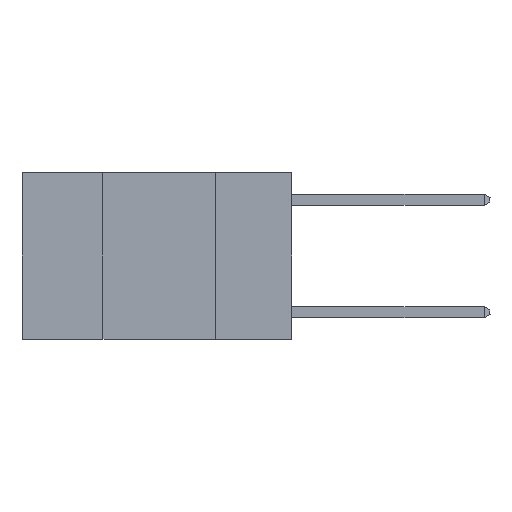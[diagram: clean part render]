
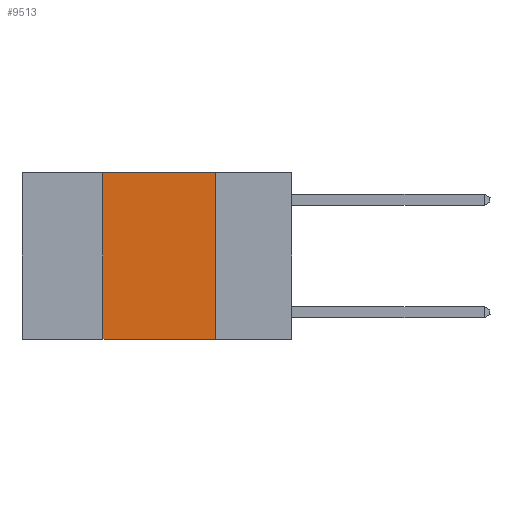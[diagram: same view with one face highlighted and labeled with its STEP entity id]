
A CAD part, left-side view. The second image highlights one B-rep face of the part: STEP entity #9513.
In plain terms, the highlighted planar face has unit normal (-1, 0, 0).
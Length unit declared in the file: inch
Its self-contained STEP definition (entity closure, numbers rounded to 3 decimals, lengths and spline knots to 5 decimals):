
#727 = DIRECTION ( 'NONE',  ( 0., -1., 0. ) ) ;
#1041 = EDGE_CURVE ( 'NONE', #17680, #10408, #16297, .T. ) ;
#2102 = LINE ( 'NONE', #2199, #7291 ) ;
#2199 = CARTESIAN_POINT ( 'NONE',  ( 0., 0.6, -0.37 ) ) ;
#2497 = CARTESIAN_POINT ( 'NONE',  ( 0., 0.17, 0. ) ) ;
#3103 = CARTESIAN_POINT ( 'NONE',  ( 0., 0.17, -0.37 ) ) ;
#3481 = VECTOR ( 'NONE', #14692, 39.37008 ) ;
#4876 = DIRECTION ( 'NONE',  ( 1., 0., 0. ) ) ;
#6159 = VECTOR ( 'NONE', #11983, 39.37008 ) ;
#6513 = VERTEX_POINT ( 'NONE', #3103 ) ;
#6905 = EDGE_CURVE ( 'NONE', #17103, #6513, #19208, .T. ) ;
#7291 = VECTOR ( 'NONE', #727, 39.37008 ) ;
#8027 = EDGE_CURVE ( 'NONE', #17680, #6513, #2102, .T. ) ;
#8838 = ORIENTED_EDGE ( 'NONE', *, *, #8027, .T. ) ;
#8993 = CARTESIAN_POINT ( 'NONE',  ( 0., 0.42, 0. ) ) ;
#9394 = AXIS2_PLACEMENT_3D ( 'NONE', #15387, #4876, #15486 ) ;
#9513 = ADVANCED_FACE ( 'NONE', ( #10910 ), #10608, .F. ) ;
#9606 = CARTESIAN_POINT ( 'NONE',  ( 0., 0.6, 0. ) ) ;
#10408 = VERTEX_POINT ( 'NONE', #14756 ) ;
#10608 = PLANE ( 'NONE',  #9394 ) ;
#10910 = FACE_OUTER_BOUND ( 'NONE', #18467, .T. ) ;
#10998 = EDGE_CURVE ( 'NONE', #10408, #17103, #18998, .T. ) ;
#11983 = DIRECTION ( 'NONE',  ( 0., 0., 1. ) ) ;
#14692 = DIRECTION ( 'NONE',  ( 0., 0., -1. ) ) ;
#14756 = CARTESIAN_POINT ( 'NONE',  ( 0., 0.42, 0. ) ) ;
#15387 = CARTESIAN_POINT ( 'NONE',  ( 0., 0.6, 0. ) ) ;
#15486 = DIRECTION ( 'NONE',  ( 0., 0., -1. ) ) ;
#15696 = CARTESIAN_POINT ( 'NONE',  ( 0., 0.17, 0. ) ) ;
#16297 = LINE ( 'NONE', #8993, #6159 ) ;
#16801 = ORIENTED_EDGE ( 'NONE', *, *, #6905, .F. ) ;
#17103 = VERTEX_POINT ( 'NONE', #15696 ) ;
#17112 = ORIENTED_EDGE ( 'NONE', *, *, #10998, .F. ) ;
#17509 = ORIENTED_EDGE ( 'NONE', *, *, #1041, .F. ) ;
#17680 = VERTEX_POINT ( 'NONE', #19466 ) ;
#18306 = VECTOR ( 'NONE', #18804, 39.37008 ) ;
#18467 = EDGE_LOOP ( 'NONE', ( #16801, #17112, #17509, #8838 ) ) ;
#18804 = DIRECTION ( 'NONE',  ( 0., -1., 0. ) ) ;
#18998 = LINE ( 'NONE', #9606, #18306 ) ;
#19208 = LINE ( 'NONE', #2497, #3481 ) ;
#19466 = CARTESIAN_POINT ( 'NONE',  ( 0., 0.42, -0.37 ) ) ;
